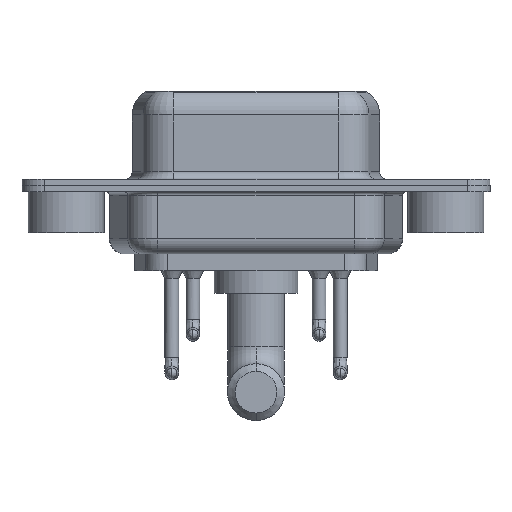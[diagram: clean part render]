
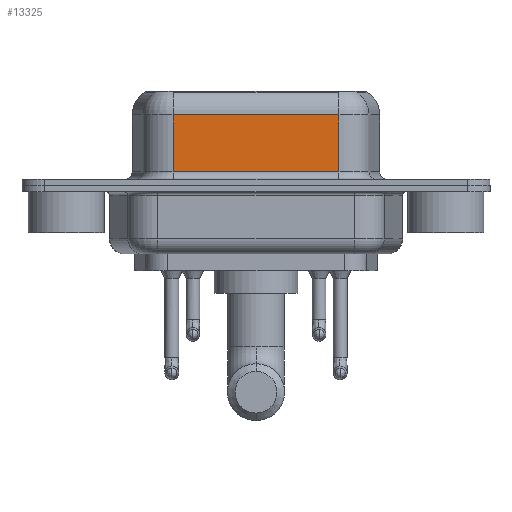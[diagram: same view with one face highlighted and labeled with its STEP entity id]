
A CAD part, front view. The second image highlights one B-rep face of the part: STEP entity #13325.
In plain terms, the highlighted planar face has unit normal (0, -1, 0).
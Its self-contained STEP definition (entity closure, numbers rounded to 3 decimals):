
#878 = DIRECTION ( 'NONE',  ( 1., 0., 0. ) ) ;
#1206 = VECTOR ( 'NONE', #6968, 1000. ) ;
#1332 = DIRECTION ( 'NONE',  ( -1., 0., 0. ) ) ;
#3734 = DIRECTION ( 'NONE',  ( -1., 0., 0. ) ) ;
#3876 = EDGE_CURVE ( 'NONE', #15465, #4791, #13010, .T. ) ;
#4730 = ORIENTED_EDGE ( 'NONE', *, *, #14064, .T. ) ;
#4762 = CARTESIAN_POINT ( 'NONE',  ( 7.038, -3.95, 4.65 ) ) ;
#4773 = CARTESIAN_POINT ( 'NONE',  ( 17.962, -3.95, 0.9 ) ) ;
#4791 = VERTEX_POINT ( 'NONE', #14358 ) ;
#5325 = LINE ( 'NONE', #7591, #9063 ) ;
#5492 = CARTESIAN_POINT ( 'NONE',  ( 17.962, -3.95, 4.65 ) ) ;
#5978 = VECTOR ( 'NONE', #878, 1000. ) ;
#6009 = LINE ( 'NONE', #12151, #5978 ) ;
#6428 = ORIENTED_EDGE ( 'NONE', *, *, #12152, .T. ) ;
#6779 = CARTESIAN_POINT ( 'NONE',  ( 7.038, -3.95, 6.4 ) ) ;
#6890 = LINE ( 'NONE', #13040, #1206 ) ;
#6968 = DIRECTION ( 'NONE',  ( 0., 0., -1. ) ) ;
#7591 = CARTESIAN_POINT ( 'NONE',  ( 17.962, -3.95, 4.65 ) ) ;
#8088 = VERTEX_POINT ( 'NONE', #5492 ) ;
#9063 = VECTOR ( 'NONE', #1332, 1000. ) ;
#9492 = VERTEX_POINT ( 'NONE', #4773 ) ;
#9891 = CARTESIAN_POINT ( 'NONE',  ( 17.962, -3.95, 6.4 ) ) ;
#11787 = DIRECTION ( 'NONE',  ( 0., 0., -1. ) ) ;
#12107 = ORIENTED_EDGE ( 'NONE', *, *, #3876, .T. ) ;
#12151 = CARTESIAN_POINT ( 'NONE',  ( 17.962, -3.95, 0.9 ) ) ;
#12152 = EDGE_CURVE ( 'NONE', #8088, #15465, #5325, .T. ) ;
#12357 = FACE_OUTER_BOUND ( 'NONE', #15130, .T. ) ;
#13010 = LINE ( 'NONE', #6779, #15694 ) ;
#13040 = CARTESIAN_POINT ( 'NONE',  ( 17.962, -3.95, 6.4 ) ) ;
#13173 = EDGE_CURVE ( 'NONE', #8088, #9492, #6890, .T. ) ;
#13325 = ADVANCED_FACE ( 'NONE', ( #12357 ), #13497, .F. ) ;
#13497 = PLANE ( 'NONE',  #15918 ) ;
#14064 = EDGE_CURVE ( 'NONE', #4791, #9492, #6009, .T. ) ;
#14358 = CARTESIAN_POINT ( 'NONE',  ( 7.038, -3.95, 0.9 ) ) ;
#14907 = DIRECTION ( 'NONE',  ( 0., 1., 0. ) ) ;
#15130 = EDGE_LOOP ( 'NONE', ( #15929, #6428, #12107, #4730 ) ) ;
#15465 = VERTEX_POINT ( 'NONE', #4762 ) ;
#15694 = VECTOR ( 'NONE', #11787, 1000. ) ;
#15918 = AXIS2_PLACEMENT_3D ( 'NONE', #9891, #14907, #3734 ) ;
#15929 = ORIENTED_EDGE ( 'NONE', *, *, #13173, .F. ) ;
